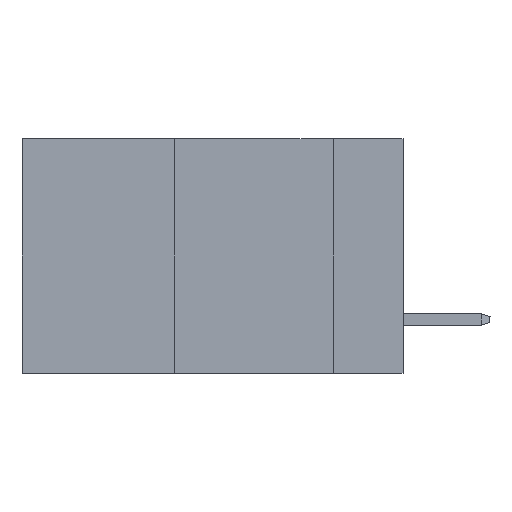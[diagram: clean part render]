
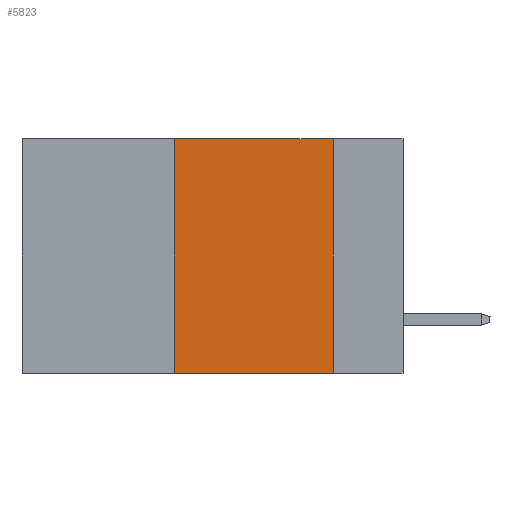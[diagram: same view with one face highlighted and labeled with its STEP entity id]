
A CAD part, left-side view. The second image highlights one B-rep face of the part: STEP entity #5823.
In plain terms, the highlighted planar face has unit normal (-1, 0, 0).
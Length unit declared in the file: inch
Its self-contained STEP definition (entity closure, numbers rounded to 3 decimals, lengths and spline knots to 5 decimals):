
#405 = LINE ( 'NONE', #509, #2960 ) ;
#509 = CARTESIAN_POINT ( 'NONE',  ( 0., 0.6, 0. ) ) ;
#729 = AXIS2_PLACEMENT_3D ( 'NONE', #20788, #20919, #5740 ) ;
#1513 = VECTOR ( 'NONE', #2424, 39.37008 ) ;
#2268 = VECTOR ( 'NONE', #8494, 39.37008 ) ;
#2424 = DIRECTION ( 'NONE',  ( 0., 0., -1. ) ) ;
#2593 = CARTESIAN_POINT ( 'NONE',  ( 0., 0.36, 0. ) ) ;
#2737 = EDGE_CURVE ( 'NONE', #8148, #17672, #18658, .T. ) ;
#2960 = VECTOR ( 'NONE', #11921, 39.37008 ) ;
#5740 = DIRECTION ( 'NONE',  ( 0., 0., -1. ) ) ;
#5823 = ADVANCED_FACE ( 'NONE', ( #12402 ), #14416, .F. ) ;
#7571 = ORIENTED_EDGE ( 'NONE', *, *, #17189, .F. ) ;
#8148 = VERTEX_POINT ( 'NONE', #18629 ) ;
#8265 = VERTEX_POINT ( 'NONE', #15429 ) ;
#8494 = DIRECTION ( 'NONE',  ( 0., 0., 1. ) ) ;
#8664 = LINE ( 'NONE', #13671, #14886 ) ;
#11921 = DIRECTION ( 'NONE',  ( 0., -1., 0. ) ) ;
#12039 = CARTESIAN_POINT ( 'NONE',  ( 0., 0.36, 0. ) ) ;
#12103 = DIRECTION ( 'NONE',  ( 0., -1., 0. ) ) ;
#12402 = FACE_OUTER_BOUND ( 'NONE', #16223, .T. ) ;
#12902 = ORIENTED_EDGE ( 'NONE', *, *, #2737, .F. ) ;
#13671 = CARTESIAN_POINT ( 'NONE',  ( 0., 0.6, -0.37 ) ) ;
#13888 = EDGE_CURVE ( 'NONE', #16130, #8265, #14176, .T. ) ;
#14176 = LINE ( 'NONE', #17580, #1513 ) ;
#14416 = PLANE ( 'NONE',  #729 ) ;
#14886 = VECTOR ( 'NONE', #12103, 39.37008 ) ;
#15429 = CARTESIAN_POINT ( 'NONE',  ( 0., 0.11, -0.37 ) ) ;
#16130 = VERTEX_POINT ( 'NONE', #18211 ) ;
#16223 = EDGE_LOOP ( 'NONE', ( #21586, #7571, #12902, #19904 ) ) ;
#17189 = EDGE_CURVE ( 'NONE', #17672, #16130, #405, .T. ) ;
#17580 = CARTESIAN_POINT ( 'NONE',  ( 0., 0.11, 0. ) ) ;
#17672 = VERTEX_POINT ( 'NONE', #2593 ) ;
#18211 = CARTESIAN_POINT ( 'NONE',  ( 0., 0.11, 0. ) ) ;
#18629 = CARTESIAN_POINT ( 'NONE',  ( 0., 0.36, -0.37 ) ) ;
#18658 = LINE ( 'NONE', #12039, #2268 ) ;
#19904 = ORIENTED_EDGE ( 'NONE', *, *, #20606, .T. ) ;
#20606 = EDGE_CURVE ( 'NONE', #8148, #8265, #8664, .T. ) ;
#20788 = CARTESIAN_POINT ( 'NONE',  ( 0., 0.6, 0. ) ) ;
#20919 = DIRECTION ( 'NONE',  ( 1., 0., 0. ) ) ;
#21586 = ORIENTED_EDGE ( 'NONE', *, *, #13888, .F. ) ;
